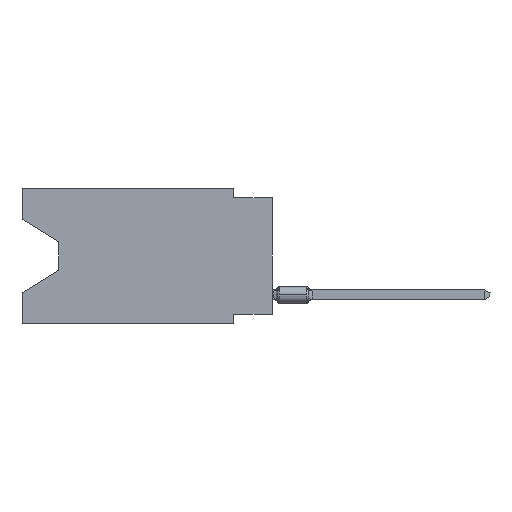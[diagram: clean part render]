
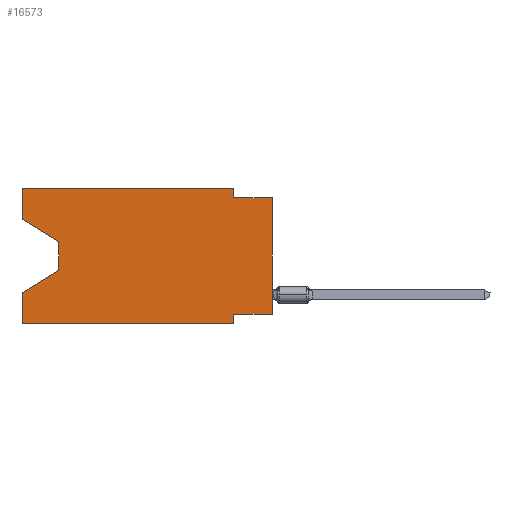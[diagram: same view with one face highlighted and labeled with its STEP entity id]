
A CAD part, left-side view. The second image highlights one B-rep face of the part: STEP entity #16573.
In plain terms, the highlighted planar face has unit normal (-1, 0, 0).
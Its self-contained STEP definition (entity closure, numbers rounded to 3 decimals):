
#990 = LINE ( 'NONE', #55083, #41668 ) ;
#2391 = DIRECTION ( 'NONE',  ( 0., 0., -1. ) ) ;
#2732 = ORIENTED_EDGE ( 'NONE', *, *, #59711, .F. ) ;
#3048 = DIRECTION ( 'NONE',  ( 0., 0., 1. ) ) ;
#4380 = EDGE_CURVE ( 'NONE', #49336, #4731, #19238, .T. ) ;
#4471 = CARTESIAN_POINT ( 'NONE',  ( 0., 16.383, -2.038 ) ) ;
#4692 = VERTEX_POINT ( 'NONE', #16973 ) ;
#4731 = VERTEX_POINT ( 'NONE', #63042 ) ;
#5367 = VERTEX_POINT ( 'NONE', #32102 ) ;
#5507 = VECTOR ( 'NONE', #52227, 1000. ) ;
#5665 = VERTEX_POINT ( 'NONE', #26389 ) ;
#6095 = ORIENTED_EDGE ( 'NONE', *, *, #42047, .F. ) ;
#6547 = CARTESIAN_POINT ( 'NONE',  ( 0., 0., -0.635 ) ) ;
#7338 = ORIENTED_EDGE ( 'NONE', *, *, #23223, .F. ) ;
#8523 = ORIENTED_EDGE ( 'NONE', *, *, #20391, .F. ) ;
#11920 = EDGE_CURVE ( 'NONE', #4731, #49173, #27251, .T. ) ;
#13174 = LINE ( 'NONE', #56099, #32643 ) ;
#14277 = VERTEX_POINT ( 'NONE', #28413 ) ;
#15656 = EDGE_LOOP ( 'NONE', ( #19039, #58018, #29503, #7338, #34545, #6095, #2732, #56592, #48541, #63304, #60100, #8523 ) ) ;
#16145 = CARTESIAN_POINT ( 'NONE',  ( 0., 16.383, -6.852 ) ) ;
#16573 = ADVANCED_FACE ( 'NONE', ( #52906 ), #48433, .F. ) ;
#16973 = CARTESIAN_POINT ( 'NONE',  ( 0., 0., -8.255 ) ) ;
#17978 = DIRECTION ( 'NONE',  ( 0., 0., 1. ) ) ;
#19039 = ORIENTED_EDGE ( 'NONE', *, *, #47517, .T. ) ;
#19238 = LINE ( 'NONE', #52563, #56238 ) ;
#19285 = CARTESIAN_POINT ( 'NONE',  ( 0., 16.383, 0. ) ) ;
#19471 = DIRECTION ( 'NONE',  ( 0., 1., 0. ) ) ;
#20350 = LINE ( 'NONE', #34763, #39056 ) ;
#20391 = EDGE_CURVE ( 'NONE', #14277, #49336, #13174, .T. ) ;
#21498 = VERTEX_POINT ( 'NONE', #47563 ) ;
#21958 = LINE ( 'NONE', #45339, #35415 ) ;
#23223 = EDGE_CURVE ( 'NONE', #46570, #43021, #21958, .T. ) ;
#26389 = CARTESIAN_POINT ( 'NONE',  ( 0., 13.97, -5.385 ) ) ;
#26449 = EDGE_CURVE ( 'NONE', #46570, #21498, #990, .T. ) ;
#26764 = DIRECTION ( 'NONE',  ( 0., 0., 1. ) ) ;
#26828 = VERTEX_POINT ( 'NONE', #44438 ) ;
#27071 = CARTESIAN_POINT ( 'NONE',  ( 0., 16.383, 0. ) ) ;
#27251 = LINE ( 'NONE', #61851, #5507 ) ;
#28413 = CARTESIAN_POINT ( 'NONE',  ( 0., 16.383, -2.038 ) ) ;
#29503 = ORIENTED_EDGE ( 'NONE', *, *, #30519, .T. ) ;
#29657 = EDGE_CURVE ( 'NONE', #4692, #32916, #38219, .T. ) ;
#30519 = EDGE_CURVE ( 'NONE', #5665, #43021, #20350, .T. ) ;
#30797 = VECTOR ( 'NONE', #3048, 1000. ) ;
#30840 = LINE ( 'NONE', #6547, #49118 ) ;
#32102 = CARTESIAN_POINT ( 'NONE',  ( 0., 13.97, -3.505 ) ) ;
#32643 = VECTOR ( 'NONE', #17978, 1000. ) ;
#32916 = VERTEX_POINT ( 'NONE', #59366 ) ;
#33573 = LINE ( 'NONE', #4471, #50898 ) ;
#34545 = ORIENTED_EDGE ( 'NONE', *, *, #26449, .T. ) ;
#34763 = CARTESIAN_POINT ( 'NONE',  ( 0., 13.97, -5.385 ) ) ;
#35415 = VECTOR ( 'NONE', #26764, 1000. ) ;
#35421 = CARTESIAN_POINT ( 'NONE',  ( 0., 2.54, -8.89 ) ) ;
#36956 = CARTESIAN_POINT ( 'NONE',  ( 0., 13.97, -3.505 ) ) ;
#38219 = LINE ( 'NONE', #47210, #30797 ) ;
#39056 = VECTOR ( 'NONE', #59099, 1000. ) ;
#39457 = AXIS2_PLACEMENT_3D ( 'NONE', #19285, #62221, #62535 ) ;
#39812 = DIRECTION ( 'NONE',  ( 0., -1., 0. ) ) ;
#40717 = VECTOR ( 'NONE', #19471, 1000. ) ;
#41660 = VECTOR ( 'NONE', #2391, 1000. ) ;
#41668 = VECTOR ( 'NONE', #44514, 1000. ) ;
#42047 = EDGE_CURVE ( 'NONE', #26828, #21498, #45013, .T. ) ;
#43021 = VERTEX_POINT ( 'NONE', #16145 ) ;
#43368 = VECTOR ( 'NONE', #44692, 1000. ) ;
#43790 = LINE ( 'NONE', #48923, #40717 ) ;
#44438 = CARTESIAN_POINT ( 'NONE',  ( 0., 2.54, -8.255 ) ) ;
#44514 = DIRECTION ( 'NONE',  ( 0., -1., 0. ) ) ;
#44692 = DIRECTION ( 'NONE',  ( 0., 0., -1. ) ) ;
#45013 = LINE ( 'NONE', #35421, #43368 ) ;
#45339 = CARTESIAN_POINT ( 'NONE',  ( 0., 16.383, 0. ) ) ;
#46570 = VERTEX_POINT ( 'NONE', #57916 ) ;
#47210 = CARTESIAN_POINT ( 'NONE',  ( 0., 0., 0. ) ) ;
#47451 = DIRECTION ( 'NONE',  ( 0., -1., 0. ) ) ;
#47517 = EDGE_CURVE ( 'NONE', #14277, #5367, #33573, .T. ) ;
#47563 = CARTESIAN_POINT ( 'NONE',  ( 0., 2.54, -8.89 ) ) ;
#48433 = PLANE ( 'NONE',  #39457 ) ;
#48541 = ORIENTED_EDGE ( 'NONE', *, *, #53560, .F. ) ;
#48923 = CARTESIAN_POINT ( 'NONE',  ( 0., 0., -8.255 ) ) ;
#49118 = VECTOR ( 'NONE', #39812, 1000. ) ;
#49173 = VERTEX_POINT ( 'NONE', #54626 ) ;
#49336 = VERTEX_POINT ( 'NONE', #27071 ) ;
#50898 = VECTOR ( 'NONE', #53108, 1000. ) ;
#52227 = DIRECTION ( 'NONE',  ( 0., 0., -1. ) ) ;
#52563 = CARTESIAN_POINT ( 'NONE',  ( 0., 16.383, 0. ) ) ;
#52906 = FACE_OUTER_BOUND ( 'NONE', #15656, .T. ) ;
#53108 = DIRECTION ( 'NONE',  ( 0., -0.855, -0.519 ) ) ;
#53560 = EDGE_CURVE ( 'NONE', #49173, #32916, #30840, .T. ) ;
#54626 = CARTESIAN_POINT ( 'NONE',  ( 0., 2.54, -0.635 ) ) ;
#55083 = CARTESIAN_POINT ( 'NONE',  ( 0., 16.383, -8.89 ) ) ;
#56099 = CARTESIAN_POINT ( 'NONE',  ( 0., 16.383, 0. ) ) ;
#56238 = VECTOR ( 'NONE', #47451, 1000. ) ;
#56592 = ORIENTED_EDGE ( 'NONE', *, *, #29657, .T. ) ;
#57199 = EDGE_CURVE ( 'NONE', #5367, #5665, #60661, .T. ) ;
#57916 = CARTESIAN_POINT ( 'NONE',  ( 0., 16.383, -8.89 ) ) ;
#58018 = ORIENTED_EDGE ( 'NONE', *, *, #57199, .T. ) ;
#59099 = DIRECTION ( 'NONE',  ( 0., 0.855, -0.519 ) ) ;
#59366 = CARTESIAN_POINT ( 'NONE',  ( 0., 0., -0.635 ) ) ;
#59711 = EDGE_CURVE ( 'NONE', #4692, #26828, #43790, .T. ) ;
#60100 = ORIENTED_EDGE ( 'NONE', *, *, #4380, .F. ) ;
#60661 = LINE ( 'NONE', #36956, #41660 ) ;
#61851 = CARTESIAN_POINT ( 'NONE',  ( 0., 2.54, 0. ) ) ;
#62221 = DIRECTION ( 'NONE',  ( 1., 0., 0. ) ) ;
#62535 = DIRECTION ( 'NONE',  ( 0., 0., -1. ) ) ;
#63042 = CARTESIAN_POINT ( 'NONE',  ( 0., 2.54, 0. ) ) ;
#63304 = ORIENTED_EDGE ( 'NONE', *, *, #11920, .F. ) ;
